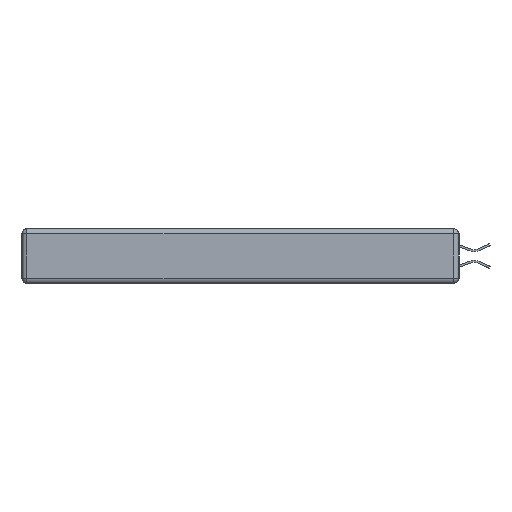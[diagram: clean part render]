
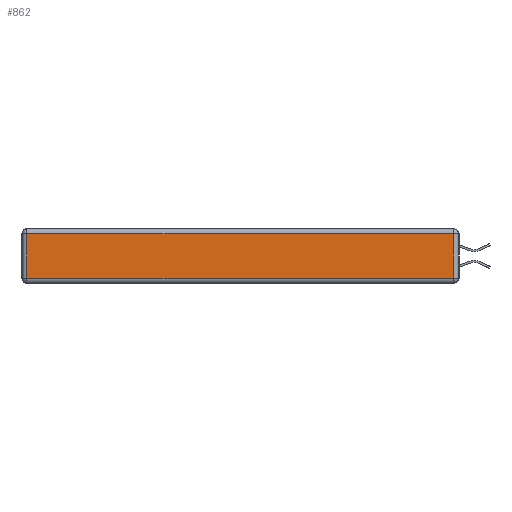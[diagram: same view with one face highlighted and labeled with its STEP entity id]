
A CAD part, left-side view. The second image highlights one B-rep face of the part: STEP entity #862.
In plain terms, the highlighted planar face has unit normal (-1, 0, 0).
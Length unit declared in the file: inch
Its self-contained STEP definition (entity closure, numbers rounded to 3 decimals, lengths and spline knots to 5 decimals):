
#862 = ADVANCED_FACE ( 'NONE', ( #23679 ), #21717, .T. ) ;
#1417 = DIRECTION ( 'NONE',  ( 0., 1., 0. ) ) ;
#2022 = VECTOR ( 'NONE', #24238, 39.37008 ) ;
#2665 = CARTESIAN_POINT ( 'NONE',  ( 0., 0., -0.313 ) ) ;
#5192 = EDGE_CURVE ( 'NONE', #23276, #16133, #16114, .T. ) ;
#5651 = AXIS2_PLACEMENT_3D ( 'NONE', #7771, #12513, #28772 ) ;
#5848 = EDGE_CURVE ( 'NONE', #13181, #23276, #15332, .T. ) ;
#5890 = VECTOR ( 'NONE', #1417, 39.37008 ) ;
#7570 = ORIENTED_EDGE ( 'NONE', *, *, #5848, .T. ) ;
#7597 = DIRECTION ( 'NONE',  ( 0., 0., 1. ) ) ;
#7771 = CARTESIAN_POINT ( 'NONE',  ( 0., 0., -0.343 ) ) ;
#9066 = CARTESIAN_POINT ( 'NONE',  ( 0., 2.72, -0.03 ) ) ;
#10164 = CARTESIAN_POINT ( 'NONE',  ( 0., 0.03, -0.343 ) ) ;
#11925 = CARTESIAN_POINT ( 'NONE',  ( 0., 2.72, -0.313 ) ) ;
#12513 = DIRECTION ( 'NONE',  ( -1., 0., 0. ) ) ;
#12651 = CARTESIAN_POINT ( 'NONE',  ( 0., 2.72, -0.343 ) ) ;
#13181 = VERTEX_POINT ( 'NONE', #18669 ) ;
#14415 = LINE ( 'NONE', #2665, #2022 ) ;
#15078 = DIRECTION ( 'NONE',  ( 0., 0., -1. ) ) ;
#15097 = ORIENTED_EDGE ( 'NONE', *, *, #25024, .T. ) ;
#15332 = LINE ( 'NONE', #10164, #27328 ) ;
#16114 = LINE ( 'NONE', #29311, #5890 ) ;
#16133 = VERTEX_POINT ( 'NONE', #9066 ) ;
#17060 = VECTOR ( 'NONE', #15078, 39.37008 ) ;
#17212 = VERTEX_POINT ( 'NONE', #11925 ) ;
#17616 = EDGE_CURVE ( 'NONE', #17212, #13181, #14415, .T. ) ;
#18669 = CARTESIAN_POINT ( 'NONE',  ( 0., 0.03, -0.313 ) ) ;
#21717 = PLANE ( 'NONE',  #5651 ) ;
#22806 = ORIENTED_EDGE ( 'NONE', *, *, #5192, .T. ) ;
#23199 = LINE ( 'NONE', #12651, #17060 ) ;
#23276 = VERTEX_POINT ( 'NONE', #24616 ) ;
#23637 = EDGE_LOOP ( 'NONE', ( #24169, #7570, #22806, #15097 ) ) ;
#23679 = FACE_OUTER_BOUND ( 'NONE', #23637, .T. ) ;
#24169 = ORIENTED_EDGE ( 'NONE', *, *, #17616, .T. ) ;
#24238 = DIRECTION ( 'NONE',  ( 0., -1., 0. ) ) ;
#24616 = CARTESIAN_POINT ( 'NONE',  ( 0., 0.03, -0.03 ) ) ;
#25024 = EDGE_CURVE ( 'NONE', #16133, #17212, #23199, .T. ) ;
#27328 = VECTOR ( 'NONE', #7597, 39.37008 ) ;
#28772 = DIRECTION ( 'NONE',  ( 0., 0., 1. ) ) ;
#29311 = CARTESIAN_POINT ( 'NONE',  ( 0., 2.75, -0.03 ) ) ;
